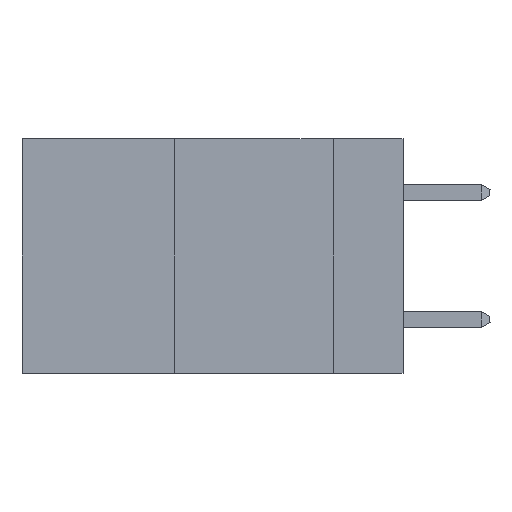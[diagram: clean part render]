
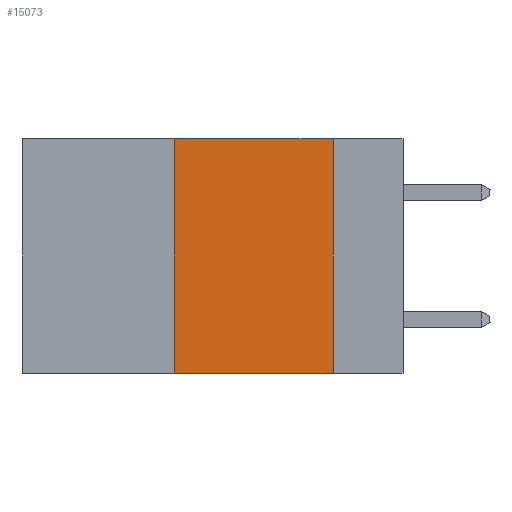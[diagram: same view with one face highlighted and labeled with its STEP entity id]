
A CAD part, left-side view. The second image highlights one B-rep face of the part: STEP entity #15073.
In plain terms, the highlighted planar face has unit normal (-1, 0, 0).
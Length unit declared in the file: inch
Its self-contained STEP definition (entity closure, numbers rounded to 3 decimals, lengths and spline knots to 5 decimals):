
#108 = ORIENTED_EDGE ( 'NONE', *, *, #3422, .T. ) ;
#1088 = CARTESIAN_POINT ( 'NONE',  ( 0., 0.36, 0. ) ) ;
#2760 = CARTESIAN_POINT ( 'NONE',  ( 0., 0.6, 0. ) ) ;
#3422 = EDGE_CURVE ( 'NONE', #11293, #24949, #12774, .T. ) ;
#4917 = ORIENTED_EDGE ( 'NONE', *, *, #26560, .F. ) ;
#7331 = PLANE ( 'NONE',  #11605 ) ;
#8813 = ORIENTED_EDGE ( 'NONE', *, *, #10683, .F. ) ;
#9104 = VECTOR ( 'NONE', #26702, 39.37008 ) ;
#9114 = CARTESIAN_POINT ( 'NONE',  ( 0., 0.11, 0. ) ) ;
#9494 = DIRECTION ( 'NONE',  ( 0., 0., -1. ) ) ;
#10683 = EDGE_CURVE ( 'NONE', #11293, #25900, #26989, .T. ) ;
#11293 = VERTEX_POINT ( 'NONE', #25098 ) ;
#11515 = CARTESIAN_POINT ( 'NONE',  ( 0., 0.6, -0.37 ) ) ;
#11605 = AXIS2_PLACEMENT_3D ( 'NONE', #22337, #19906, #9494 ) ;
#11693 = EDGE_LOOP ( 'NONE', ( #4917, #18081, #8813, #108 ) ) ;
#12774 = LINE ( 'NONE', #11515, #9104 ) ;
#13038 = EDGE_CURVE ( 'NONE', #25900, #26735, #20829, .T. ) ;
#13168 = DIRECTION ( 'NONE',  ( 0., -1., 0. ) ) ;
#13406 = CARTESIAN_POINT ( 'NONE',  ( 0., 0.11, -0.37 ) ) ;
#13509 = CARTESIAN_POINT ( 'NONE',  ( 0., 0.36, 0. ) ) ;
#15073 = ADVANCED_FACE ( 'NONE', ( #18343 ), #7331, .F. ) ;
#15572 = VECTOR ( 'NONE', #24836, 39.37008 ) ;
#18081 = ORIENTED_EDGE ( 'NONE', *, *, #13038, .F. ) ;
#18343 = FACE_OUTER_BOUND ( 'NONE', #11693, .T. ) ;
#19598 = VECTOR ( 'NONE', #22142, 39.37008 ) ;
#19823 = VECTOR ( 'NONE', #13168, 39.37008 ) ;
#19906 = DIRECTION ( 'NONE',  ( 1., 0., 0. ) ) ;
#20829 = LINE ( 'NONE', #2760, #19823 ) ;
#21621 = LINE ( 'NONE', #9114, #19598 ) ;
#22142 = DIRECTION ( 'NONE',  ( 0., 0., -1. ) ) ;
#22337 = CARTESIAN_POINT ( 'NONE',  ( 0., 0.6, 0. ) ) ;
#24836 = DIRECTION ( 'NONE',  ( 0., 0., 1. ) ) ;
#24949 = VERTEX_POINT ( 'NONE', #13406 ) ;
#25098 = CARTESIAN_POINT ( 'NONE',  ( 0., 0.36, -0.37 ) ) ;
#25900 = VERTEX_POINT ( 'NONE', #13509 ) ;
#26560 = EDGE_CURVE ( 'NONE', #26735, #24949, #21621, .T. ) ;
#26702 = DIRECTION ( 'NONE',  ( 0., -1., 0. ) ) ;
#26735 = VERTEX_POINT ( 'NONE', #26909 ) ;
#26909 = CARTESIAN_POINT ( 'NONE',  ( 0., 0.11, 0. ) ) ;
#26989 = LINE ( 'NONE', #1088, #15572 ) ;
